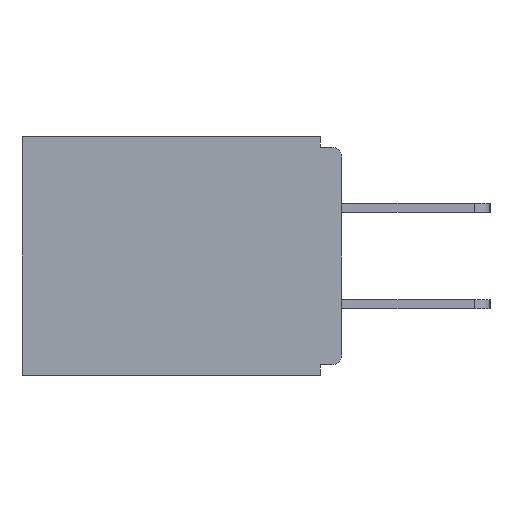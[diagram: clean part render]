
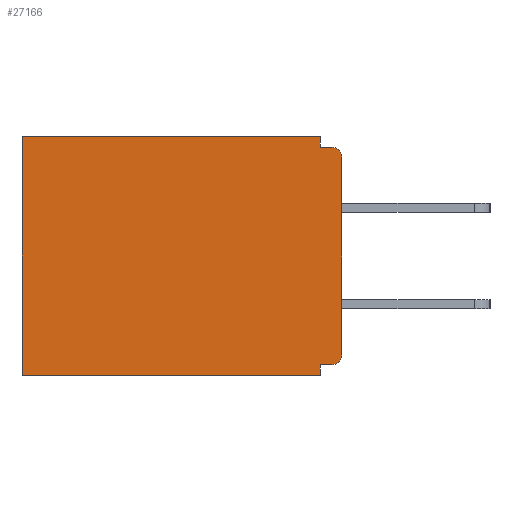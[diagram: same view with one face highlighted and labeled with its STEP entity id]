
A CAD part, left-side view. The second image highlights one B-rep face of the part: STEP entity #27166.
In plain terms, the highlighted planar face has unit normal (-1, 0, 0).
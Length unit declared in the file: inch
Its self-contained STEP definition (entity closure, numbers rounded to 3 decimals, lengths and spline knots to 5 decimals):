
#134 = VECTOR ( 'NONE', #21337, 39.37008 ) ;
#726 = EDGE_CURVE ( 'NONE', #4124, #2132, #21574, .T. ) ;
#1055 = EDGE_CURVE ( 'NONE', #14020, #9123, #22995, .T. ) ;
#1112 = DIRECTION ( 'NONE',  ( 0., 0., -1. ) ) ;
#2058 = CARTESIAN_POINT ( 'NONE',  ( 0.298, 0.015, -0.015 ) ) ;
#2077 = VERTEX_POINT ( 'NONE', #4107 ) ;
#2132 = VERTEX_POINT ( 'NONE', #27800 ) ;
#2192 = CARTESIAN_POINT ( 'NONE',  ( 0.298, 0.015, -0.328 ) ) ;
#2317 = AXIS2_PLACEMENT_3D ( 'NONE', #8553, #24767, #19871 ) ;
#2689 = AXIS2_PLACEMENT_3D ( 'NONE', #20259, #15344, #13170 ) ;
#4036 = VECTOR ( 'NONE', #20322, 39.37008 ) ;
#4107 = CARTESIAN_POINT ( 'NONE',  ( 0.298, 0.031, -0.343 ) ) ;
#4124 = VERTEX_POINT ( 'NONE', #28372 ) ;
#4244 = VERTEX_POINT ( 'NONE', #26806 ) ;
#4633 = AXIS2_PLACEMENT_3D ( 'NONE', #28621, #14895, #5691 ) ;
#4948 = CARTESIAN_POINT ( 'NONE',  ( 0.298, 0., 0. ) ) ;
#5215 = ORIENTED_EDGE ( 'NONE', *, *, #10466, .F. ) ;
#5331 = ORIENTED_EDGE ( 'NONE', *, *, #26804, .F. ) ;
#5691 = DIRECTION ( 'NONE',  ( 0., 0., -1. ) ) ;
#7809 = LINE ( 'NONE', #15478, #16761 ) ;
#7860 = LINE ( 'NONE', #21671, #28630 ) ;
#8553 = CARTESIAN_POINT ( 'NONE',  ( 0.298, 0.015, -0.03 ) ) ;
#8575 = LINE ( 'NONE', #19549, #14993 ) ;
#8601 = DIRECTION ( 'NONE',  ( 0., 1., 0. ) ) ;
#8821 = DIRECTION ( 'NONE',  ( 0., 1., 0. ) ) ;
#8835 = VERTEX_POINT ( 'NONE', #17812 ) ;
#9123 = VERTEX_POINT ( 'NONE', #28865 ) ;
#9705 = LINE ( 'NONE', #4948, #25470 ) ;
#9796 = CARTESIAN_POINT ( 'NONE',  ( 0.298, 0.031, -0.328 ) ) ;
#10301 = VECTOR ( 'NONE', #8821, 39.37008 ) ;
#10342 = DIRECTION ( 'NONE',  ( 0., -1., 0. ) ) ;
#10466 = EDGE_CURVE ( 'NONE', #14020, #24659, #7809, .T. ) ;
#12406 = PLANE ( 'NONE',  #4633 ) ;
#13170 = DIRECTION ( 'NONE',  ( 0., 0., -1. ) ) ;
#14020 = VERTEX_POINT ( 'NONE', #2192 ) ;
#14042 = EDGE_CURVE ( 'NONE', #2077, #4244, #27831, .T. ) ;
#14895 = DIRECTION ( 'NONE',  ( 1., 0., 0. ) ) ;
#14976 = FACE_OUTER_BOUND ( 'NONE', #27728, .T. ) ;
#14993 = VECTOR ( 'NONE', #10342, 39.37008 ) ;
#15344 = DIRECTION ( 'NONE',  ( -1., 0., 0. ) ) ;
#15478 = CARTESIAN_POINT ( 'NONE',  ( 0.298, 0., -0.328 ) ) ;
#15647 = EDGE_CURVE ( 'NONE', #16683, #25750, #17743, .T. ) ;
#15933 = ORIENTED_EDGE ( 'NONE', *, *, #15647, .T. ) ;
#16410 = ORIENTED_EDGE ( 'NONE', *, *, #29313, .T. ) ;
#16577 = ORIENTED_EDGE ( 'NONE', *, *, #21458, .F. ) ;
#16588 = DIRECTION ( 'NONE',  ( 0., 0., -1. ) ) ;
#16683 = VERTEX_POINT ( 'NONE', #23629 ) ;
#16761 = VECTOR ( 'NONE', #8601, 39.37008 ) ;
#16840 = EDGE_CURVE ( 'NONE', #24659, #2077, #20537, .T. ) ;
#16927 = CARTESIAN_POINT ( 'NONE',  ( 0.298, 0.031, -0.343 ) ) ;
#16998 = CARTESIAN_POINT ( 'NONE',  ( 0.298, 0.031, -0.343 ) ) ;
#17743 = CIRCLE ( 'NONE', #2317, 0.015 ) ;
#17812 = CARTESIAN_POINT ( 'NONE',  ( 0.298, 0.46, 0. ) ) ;
#17814 = ORIENTED_EDGE ( 'NONE', *, *, #16840, .F. ) ;
#17996 = ORIENTED_EDGE ( 'NONE', *, *, #14042, .F. ) ;
#18217 = CARTESIAN_POINT ( 'NONE',  ( 0.298, 0., -0.343 ) ) ;
#19010 = CARTESIAN_POINT ( 'NONE',  ( 0.298, 0.46, 0. ) ) ;
#19549 = CARTESIAN_POINT ( 'NONE',  ( 0.298, 0., -0.015 ) ) ;
#19871 = DIRECTION ( 'NONE',  ( 0., 0., -1. ) ) ;
#20259 = CARTESIAN_POINT ( 'NONE',  ( 0.298, 0.015, -0.313 ) ) ;
#20322 = DIRECTION ( 'NONE',  ( 0., 0., -1. ) ) ;
#20537 = LINE ( 'NONE', #16998, #25871 ) ;
#21337 = DIRECTION ( 'NONE',  ( 0., 0., -1. ) ) ;
#21458 = EDGE_CURVE ( 'NONE', #2132, #25750, #8575, .T. ) ;
#21574 = LINE ( 'NONE', #16927, #4036 ) ;
#21671 = CARTESIAN_POINT ( 'NONE',  ( 0.298, 0., 0. ) ) ;
#22995 = CIRCLE ( 'NONE', #2689, 0.015 ) ;
#23629 = CARTESIAN_POINT ( 'NONE',  ( 0.298, 0., -0.03 ) ) ;
#24659 = VERTEX_POINT ( 'NONE', #9796 ) ;
#24767 = DIRECTION ( 'NONE',  ( -1., 0., 0. ) ) ;
#25470 = VECTOR ( 'NONE', #27390, 39.37008 ) ;
#25750 = VERTEX_POINT ( 'NONE', #2058 ) ;
#25871 = VECTOR ( 'NONE', #16588, 39.37008 ) ;
#25889 = EDGE_CURVE ( 'NONE', #4124, #8835, #9705, .T. ) ;
#26033 = ORIENTED_EDGE ( 'NONE', *, *, #726, .F. ) ;
#26804 = EDGE_CURVE ( 'NONE', #16683, #9123, #7860, .T. ) ;
#26806 = CARTESIAN_POINT ( 'NONE',  ( 0.298, 0.46, -0.343 ) ) ;
#26989 = ORIENTED_EDGE ( 'NONE', *, *, #25889, .T. ) ;
#27166 = ADVANCED_FACE ( 'NONE', ( #14976 ), #12406, .F. ) ;
#27390 = DIRECTION ( 'NONE',  ( 0., 1., 0. ) ) ;
#27404 = LINE ( 'NONE', #19010, #134 ) ;
#27728 = EDGE_LOOP ( 'NONE', ( #15933, #16577, #26033, #26989, #16410, #17996, #17814, #5215, #28773, #5331 ) ) ;
#27800 = CARTESIAN_POINT ( 'NONE',  ( 0.298, 0.031, -0.015 ) ) ;
#27831 = LINE ( 'NONE', #18217, #10301 ) ;
#28372 = CARTESIAN_POINT ( 'NONE',  ( 0.298, 0.031, 0. ) ) ;
#28621 = CARTESIAN_POINT ( 'NONE',  ( 0.298, 0., 0. ) ) ;
#28630 = VECTOR ( 'NONE', #1112, 39.37008 ) ;
#28773 = ORIENTED_EDGE ( 'NONE', *, *, #1055, .T. ) ;
#28865 = CARTESIAN_POINT ( 'NONE',  ( 0.298, 0., -0.313 ) ) ;
#29313 = EDGE_CURVE ( 'NONE', #8835, #4244, #27404, .T. ) ;
